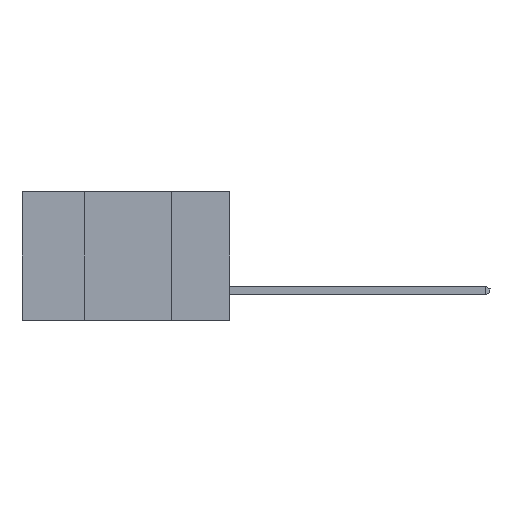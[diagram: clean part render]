
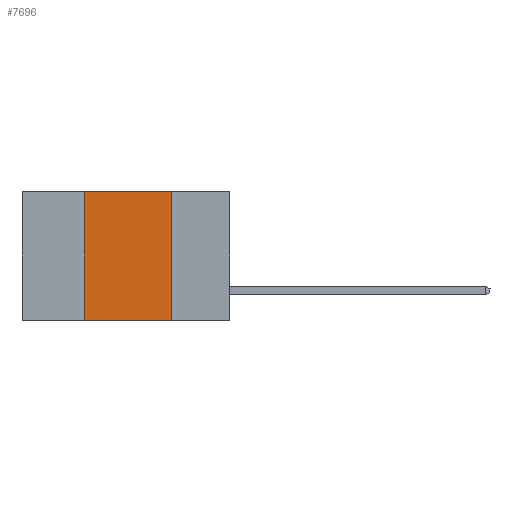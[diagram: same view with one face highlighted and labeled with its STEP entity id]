
A CAD part, left-side view. The second image highlights one B-rep face of the part: STEP entity #7696.
In plain terms, the highlighted planar face has unit normal (-1, 0, 0).
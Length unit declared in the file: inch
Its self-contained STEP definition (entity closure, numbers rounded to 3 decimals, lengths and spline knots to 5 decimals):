
#404 = PLANE ( 'NONE',  #11055 ) ;
#582 = CARTESIAN_POINT ( 'NONE',  ( 0., 0.6, -0.37 ) ) ;
#945 = VECTOR ( 'NONE', #6202, 39.37008 ) ;
#987 = LINE ( 'NONE', #10934, #6450 ) ;
#1173 = LINE ( 'NONE', #2568, #945 ) ;
#1663 = CARTESIAN_POINT ( 'NONE',  ( 0., 0.42, -0.37 ) ) ;
#2508 = EDGE_LOOP ( 'NONE', ( #10296, #12566, #3596, #12978 ) ) ;
#2568 = CARTESIAN_POINT ( 'NONE',  ( 0., 0.6, 0. ) ) ;
#2817 = EDGE_CURVE ( 'NONE', #3108, #15368, #1173, .T. ) ;
#2870 = DIRECTION ( 'NONE',  ( 0., -1., 0. ) ) ;
#3108 = VERTEX_POINT ( 'NONE', #15674 ) ;
#3516 = EDGE_CURVE ( 'NONE', #15368, #4544, #7962, .T. ) ;
#3596 = ORIENTED_EDGE ( 'NONE', *, *, #12681, .F. ) ;
#4261 = DIRECTION ( 'NONE',  ( 0., 0., -1. ) ) ;
#4544 = VERTEX_POINT ( 'NONE', #13962 ) ;
#5440 = LINE ( 'NONE', #582, #12469 ) ;
#5972 = DIRECTION ( 'NONE',  ( 0., 0., 1. ) ) ;
#6202 = DIRECTION ( 'NONE',  ( 0., -1., 0. ) ) ;
#6450 = VECTOR ( 'NONE', #5972, 39.37008 ) ;
#7696 = ADVANCED_FACE ( 'NONE', ( #7794 ), #404, .F. ) ;
#7794 = FACE_OUTER_BOUND ( 'NONE', #2508, .T. ) ;
#7962 = LINE ( 'NONE', #8208, #12768 ) ;
#8208 = CARTESIAN_POINT ( 'NONE',  ( 0., 0.17, -0.37 ) ) ;
#8236 = CARTESIAN_POINT ( 'NONE',  ( 0., 0.17, 0. ) ) ;
#10296 = ORIENTED_EDGE ( 'NONE', *, *, #3516, .F. ) ;
#10341 = CARTESIAN_POINT ( 'NONE',  ( 0., 0.6, 0. ) ) ;
#10934 = CARTESIAN_POINT ( 'NONE',  ( 0., 0.42, -0.37 ) ) ;
#11055 = AXIS2_PLACEMENT_3D ( 'NONE', #10341, #11501, #4261 ) ;
#11501 = DIRECTION ( 'NONE',  ( 1., 0., 0. ) ) ;
#12469 = VECTOR ( 'NONE', #2870, 39.37008 ) ;
#12566 = ORIENTED_EDGE ( 'NONE', *, *, #2817, .F. ) ;
#12681 = EDGE_CURVE ( 'NONE', #15477, #3108, #987, .T. ) ;
#12768 = VECTOR ( 'NONE', #12962, 39.37008 ) ;
#12962 = DIRECTION ( 'NONE',  ( 0., 0., -1. ) ) ;
#12978 = ORIENTED_EDGE ( 'NONE', *, *, #14355, .T. ) ;
#13962 = CARTESIAN_POINT ( 'NONE',  ( 0., 0.17, -0.37 ) ) ;
#14355 = EDGE_CURVE ( 'NONE', #15477, #4544, #5440, .T. ) ;
#15368 = VERTEX_POINT ( 'NONE', #8236 ) ;
#15477 = VERTEX_POINT ( 'NONE', #1663 ) ;
#15674 = CARTESIAN_POINT ( 'NONE',  ( 0., 0.42, 0. ) ) ;
